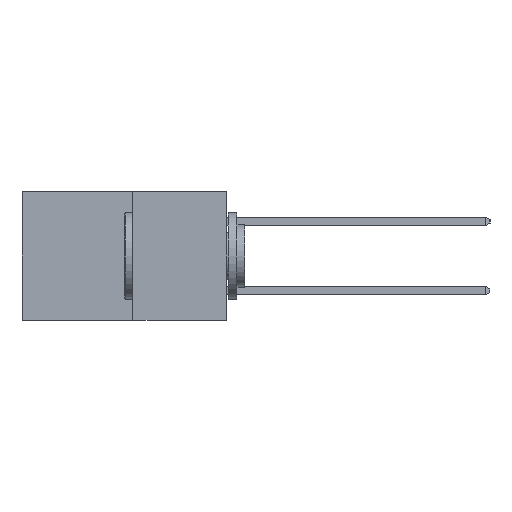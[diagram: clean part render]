
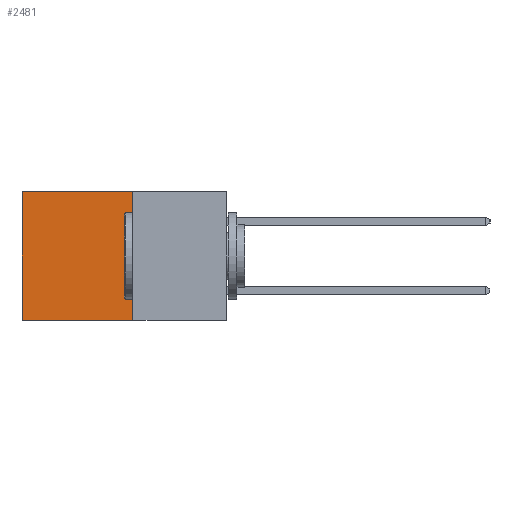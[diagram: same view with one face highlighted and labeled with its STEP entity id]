
A CAD part, left-side view. The second image highlights one B-rep face of the part: STEP entity #2481.
In plain terms, the highlighted planar face has unit normal (-1, 0, 0).
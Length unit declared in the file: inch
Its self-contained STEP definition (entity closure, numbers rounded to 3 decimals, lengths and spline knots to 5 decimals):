
#52 = ORIENTED_EDGE ( 'NONE', *, *, #3375, .T. ) ;
#128 = LINE ( 'NONE', #7081, #2254 ) ;
#287 = DIRECTION ( 'NONE',  ( 1., 0., 0. ) ) ;
#308 = DIRECTION ( 'NONE',  ( 0., 0., -1. ) ) ;
#420 = ORIENTED_EDGE ( 'NONE', *, *, #8247, .T. ) ;
#435 = VECTOR ( 'NONE', #8255, 39.37008 ) ;
#529 = CARTESIAN_POINT ( 'NONE',  ( 0.277, 0.27, -0.37 ) ) ;
#952 = PLANE ( 'NONE',  #8191 ) ;
#1017 = CARTESIAN_POINT ( 'NONE',  ( 0.277, 0.59, -0.37 ) ) ;
#1128 = EDGE_CURVE ( 'NONE', #6975, #9304, #8351, .T. ) ;
#1982 = CARTESIAN_POINT ( 'NONE',  ( 0.277, 0.27, 0. ) ) ;
#2254 = VECTOR ( 'NONE', #7025, 39.37008 ) ;
#2397 = CARTESIAN_POINT ( 'NONE',  ( 0.277, 0.59, 0. ) ) ;
#2433 = FACE_OUTER_BOUND ( 'NONE', #3705, .T. ) ;
#2481 = ADVANCED_FACE ( 'NONE', ( #2433 ), #952, .F. ) ;
#2489 = CARTESIAN_POINT ( 'NONE',  ( 0.277, 0.27, 0. ) ) ;
#2617 = LINE ( 'NONE', #4458, #435 ) ;
#3375 = EDGE_CURVE ( 'NONE', #9458, #8430, #128, .T. ) ;
#3398 = DIRECTION ( 'NONE',  ( 0., 1., 0. ) ) ;
#3705 = EDGE_LOOP ( 'NONE', ( #52, #6496, #8605, #420 ) ) ;
#4458 = CARTESIAN_POINT ( 'NONE',  ( 0.277, 0.27, -0.37 ) ) ;
#4523 = CARTESIAN_POINT ( 'NONE',  ( 0.277, 0.27, -0.37 ) ) ;
#6048 = EDGE_CURVE ( 'NONE', #9304, #8430, #2617, .T. ) ;
#6293 = CARTESIAN_POINT ( 'NONE',  ( 0.277, 0.27, -0.37 ) ) ;
#6328 = VECTOR ( 'NONE', #9751, 39.37008 ) ;
#6496 = ORIENTED_EDGE ( 'NONE', *, *, #6048, .F. ) ;
#6961 = VECTOR ( 'NONE', #3398, 39.37008 ) ;
#6975 = VERTEX_POINT ( 'NONE', #1982 ) ;
#7025 = DIRECTION ( 'NONE',  ( 0., 0., -1. ) ) ;
#7081 = CARTESIAN_POINT ( 'NONE',  ( 0.277, 0.59, -0.37 ) ) ;
#7428 = LINE ( 'NONE', #2489, #6961 ) ;
#8191 = AXIS2_PLACEMENT_3D ( 'NONE', #4523, #287, #308 ) ;
#8247 = EDGE_CURVE ( 'NONE', #6975, #9458, #7428, .T. ) ;
#8255 = DIRECTION ( 'NONE',  ( 0., 1., 0. ) ) ;
#8351 = LINE ( 'NONE', #529, #6328 ) ;
#8430 = VERTEX_POINT ( 'NONE', #1017 ) ;
#8605 = ORIENTED_EDGE ( 'NONE', *, *, #1128, .F. ) ;
#9304 = VERTEX_POINT ( 'NONE', #6293 ) ;
#9458 = VERTEX_POINT ( 'NONE', #2397 ) ;
#9751 = DIRECTION ( 'NONE',  ( 0., 0., -1. ) ) ;
